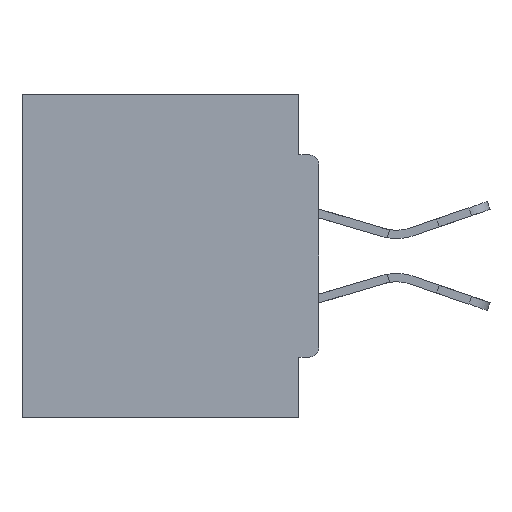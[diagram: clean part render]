
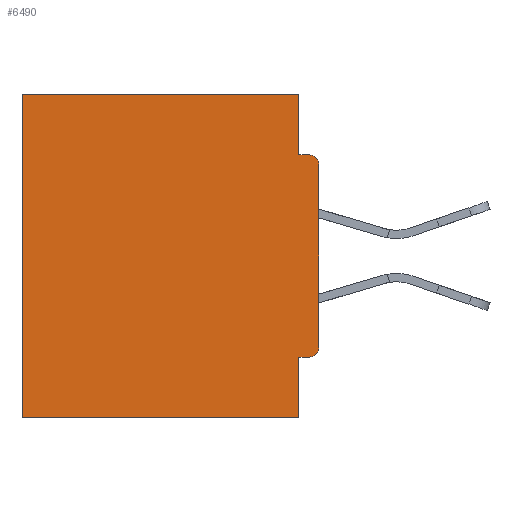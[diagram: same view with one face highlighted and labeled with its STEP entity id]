
A CAD part, left-side view. The second image highlights one B-rep face of the part: STEP entity #6490.
In plain terms, the highlighted planar face has unit normal (-1, 0, 0).
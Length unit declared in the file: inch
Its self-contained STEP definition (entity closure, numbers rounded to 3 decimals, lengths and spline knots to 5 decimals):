
#154 = CARTESIAN_POINT ( 'NONE',  ( 0.298, 0.031, -0.0935 ) ) ;
#1057 = CARTESIAN_POINT ( 'NONE',  ( 0.298, 0.015, -0.4065 ) ) ;
#1341 = DIRECTION ( 'NONE',  ( 0., 1., 0. ) ) ;
#1554 = VERTEX_POINT ( 'NONE', #1057 ) ;
#1675 = DIRECTION ( 'NONE',  ( 0., 0., -1. ) ) ;
#1699 = CARTESIAN_POINT ( 'NONE',  ( 0.298, 0.015, -0.1085 ) ) ;
#2545 = CARTESIAN_POINT ( 'NONE',  ( 0.298, 0.46, -0.5 ) ) ;
#3037 = FACE_OUTER_BOUND ( 'NONE', #22324, .T. ) ;
#3533 = PLANE ( 'NONE',  #4271 ) ;
#4172 = CARTESIAN_POINT ( 'NONE',  ( 0.298, 0., -0.1085 ) ) ;
#4266 = DIRECTION ( 'NONE',  ( -1., 0., 0. ) ) ;
#4271 = AXIS2_PLACEMENT_3D ( 'NONE', #10293, #36780, #10421 ) ;
#5116 = EDGE_CURVE ( 'NONE', #18499, #29337, #14785, .T. ) ;
#5119 = CARTESIAN_POINT ( 'NONE',  ( 0.298, 0., -0.3915 ) ) ;
#5270 = EDGE_CURVE ( 'NONE', #7075, #29337, #14757, .T. ) ;
#5957 = CARTESIAN_POINT ( 'NONE',  ( 0.298, 0.46, 0. ) ) ;
#6076 = DIRECTION ( 'NONE',  ( 0., 0., -1. ) ) ;
#6166 = LINE ( 'NONE', #23929, #21314 ) ;
#6490 = ADVANCED_FACE ( 'NONE', ( #3037 ), #3533, .F. ) ;
#7075 = VERTEX_POINT ( 'NONE', #30296 ) ;
#7544 = VERTEX_POINT ( 'NONE', #22174 ) ;
#8148 = ORIENTED_EDGE ( 'NONE', *, *, #8919, .T. ) ;
#8919 = EDGE_CURVE ( 'NONE', #1554, #19376, #27641, .T. ) ;
#10036 = LINE ( 'NONE', #18813, #26138 ) ;
#10197 = CARTESIAN_POINT ( 'NONE',  ( 0.298, 0., -0.5 ) ) ;
#10293 = CARTESIAN_POINT ( 'NONE',  ( 0.298, 0., 0. ) ) ;
#10421 = DIRECTION ( 'NONE',  ( 0., 0., -1. ) ) ;
#10654 = VERTEX_POINT ( 'NONE', #154 ) ;
#11993 = CARTESIAN_POINT ( 'NONE',  ( 0.298, 0.031, -0.5 ) ) ;
#12702 = ORIENTED_EDGE ( 'NONE', *, *, #29976, .T. ) ;
#12736 = CARTESIAN_POINT ( 'NONE',  ( 0.298, 0., -0.0935 ) ) ;
#13293 = VERTEX_POINT ( 'NONE', #31053 ) ;
#14108 = DIRECTION ( 'NONE',  ( 0., 1., 0. ) ) ;
#14757 = LINE ( 'NONE', #5957, #37328 ) ;
#14785 = LINE ( 'NONE', #10197, #22103 ) ;
#15195 = DIRECTION ( 'NONE',  ( 0., 0., -1. ) ) ;
#15236 = LINE ( 'NONE', #33002, #29480 ) ;
#15300 = LINE ( 'NONE', #11993, #32773 ) ;
#16165 = LINE ( 'NONE', #12736, #30005 ) ;
#16228 = LINE ( 'NONE', #30848, #31913 ) ;
#16471 = ORIENTED_EDGE ( 'NONE', *, *, #5270, .T. ) ;
#16786 = DIRECTION ( 'NONE',  ( 0., 0., -1. ) ) ;
#18149 = ORIENTED_EDGE ( 'NONE', *, *, #18577, .F. ) ;
#18499 = VERTEX_POINT ( 'NONE', #26875 ) ;
#18522 = ORIENTED_EDGE ( 'NONE', *, *, #26531, .F. ) ;
#18577 = EDGE_CURVE ( 'NONE', #13293, #18499, #15300, .T. ) ;
#18638 = EDGE_CURVE ( 'NONE', #10654, #28093, #16165, .T. ) ;
#18813 = CARTESIAN_POINT ( 'NONE',  ( 0.298, 0., -0.4065 ) ) ;
#19265 = EDGE_CURVE ( 'NONE', #24842, #19376, #15236, .T. ) ;
#19376 = VERTEX_POINT ( 'NONE', #5119 ) ;
#19788 = DIRECTION ( 'NONE',  ( -1., 0., 0. ) ) ;
#20176 = ORIENTED_EDGE ( 'NONE', *, *, #18638, .F. ) ;
#20645 = ORIENTED_EDGE ( 'NONE', *, *, #31472, .F. ) ;
#21314 = VECTOR ( 'NONE', #15195, 39.37008 ) ;
#21455 = DIRECTION ( 'NONE',  ( 0., -1., 0. ) ) ;
#22103 = VECTOR ( 'NONE', #1341, 39.37008 ) ;
#22174 = CARTESIAN_POINT ( 'NONE',  ( 0.298, 0.031, 0. ) ) ;
#22216 = AXIS2_PLACEMENT_3D ( 'NONE', #31360, #19788, #16786 ) ;
#22324 = EDGE_LOOP ( 'NONE', ( #36295, #20176, #20645, #12702, #16471, #23469, #18149, #18522, #8148, #33419 ) ) ;
#23469 = ORIENTED_EDGE ( 'NONE', *, *, #5116, .F. ) ;
#23929 = CARTESIAN_POINT ( 'NONE',  ( 0.298, 0.031, -0.5 ) ) ;
#23971 = CARTESIAN_POINT ( 'NONE',  ( 0.298, 0.015, -0.0935 ) ) ;
#24466 = DIRECTION ( 'NONE',  ( 0., 1., 0. ) ) ;
#24529 = DIRECTION ( 'NONE',  ( 0., 0., -1. ) ) ;
#24842 = VERTEX_POINT ( 'NONE', #4172 ) ;
#25271 = CIRCLE ( 'NONE', #25728, 0.015 ) ;
#25728 = AXIS2_PLACEMENT_3D ( 'NONE', #1699, #4266, #1675 ) ;
#26138 = VECTOR ( 'NONE', #24466, 39.37008 ) ;
#26531 = EDGE_CURVE ( 'NONE', #1554, #13293, #10036, .T. ) ;
#26875 = CARTESIAN_POINT ( 'NONE',  ( 0.298, 0.031, -0.5 ) ) ;
#26948 = DIRECTION ( 'NONE',  ( 0., 0., -1. ) ) ;
#27641 = CIRCLE ( 'NONE', #22216, 0.015 ) ;
#28093 = VERTEX_POINT ( 'NONE', #23971 ) ;
#29337 = VERTEX_POINT ( 'NONE', #2545 ) ;
#29480 = VECTOR ( 'NONE', #26948, 39.37008 ) ;
#29976 = EDGE_CURVE ( 'NONE', #7544, #7075, #16228, .T. ) ;
#30005 = VECTOR ( 'NONE', #21455, 39.37008 ) ;
#30296 = CARTESIAN_POINT ( 'NONE',  ( 0.298, 0.46, 0. ) ) ;
#30848 = CARTESIAN_POINT ( 'NONE',  ( 0.298, 0., 0. ) ) ;
#31053 = CARTESIAN_POINT ( 'NONE',  ( 0.298, 0.031, -0.4065 ) ) ;
#31360 = CARTESIAN_POINT ( 'NONE',  ( 0.298, 0.015, -0.3915 ) ) ;
#31472 = EDGE_CURVE ( 'NONE', #7544, #10654, #6166, .T. ) ;
#31913 = VECTOR ( 'NONE', #14108, 39.37008 ) ;
#32773 = VECTOR ( 'NONE', #24529, 39.37008 ) ;
#33002 = CARTESIAN_POINT ( 'NONE',  ( 0.298, 0., 0. ) ) ;
#33419 = ORIENTED_EDGE ( 'NONE', *, *, #19265, .F. ) ;
#33516 = EDGE_CURVE ( 'NONE', #24842, #28093, #25271, .T. ) ;
#36295 = ORIENTED_EDGE ( 'NONE', *, *, #33516, .T. ) ;
#36780 = DIRECTION ( 'NONE',  ( 1., 0., 0. ) ) ;
#37328 = VECTOR ( 'NONE', #6076, 39.37008 ) ;
